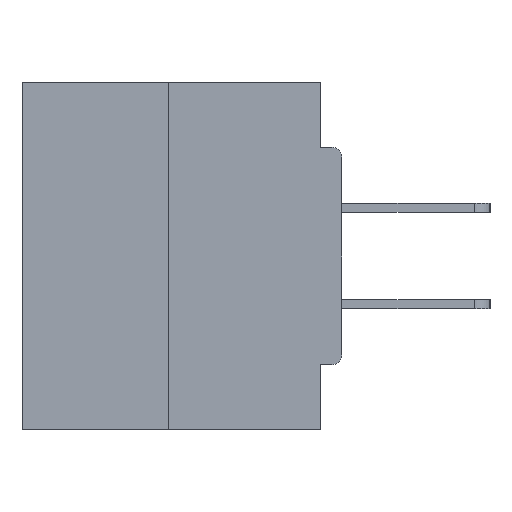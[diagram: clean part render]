
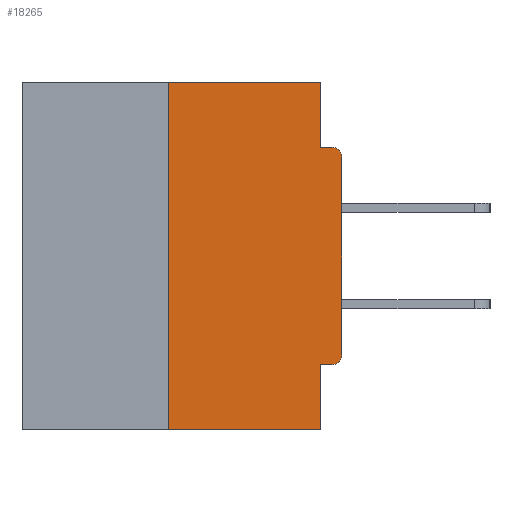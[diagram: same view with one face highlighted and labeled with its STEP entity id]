
A CAD part, left-side view. The second image highlights one B-rep face of the part: STEP entity #18265.
In plain terms, the highlighted planar face has unit normal (-1, 0, 0).
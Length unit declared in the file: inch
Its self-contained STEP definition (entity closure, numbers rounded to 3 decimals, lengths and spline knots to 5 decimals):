
#189 = CIRCLE ( 'NONE', #26565, 0.015 ) ;
#713 = DIRECTION ( 'NONE',  ( 0., -1., 0. ) ) ;
#1690 = CARTESIAN_POINT ( 'NONE',  ( 0., 0.25, 0. ) ) ;
#2110 = CARTESIAN_POINT ( 'NONE',  ( 0., 0.015, -0.0935 ) ) ;
#2321 = PLANE ( 'NONE',  #33226 ) ;
#3088 = EDGE_CURVE ( 'NONE', #15137, #19383, #21473, .T. ) ;
#3170 = VECTOR ( 'NONE', #7702, 39.37008 ) ;
#3709 = EDGE_CURVE ( 'NONE', #34003, #10903, #13700, .T. ) ;
#3812 = LINE ( 'NONE', #26926, #5011 ) ;
#3874 = FACE_OUTER_BOUND ( 'NONE', #22107, .T. ) ;
#4097 = VERTEX_POINT ( 'NONE', #36833 ) ;
#5011 = VECTOR ( 'NONE', #15619, 39.37008 ) ;
#5798 = ORIENTED_EDGE ( 'NONE', *, *, #3088, .T. ) ;
#5903 = CARTESIAN_POINT ( 'NONE',  ( 0., 0.031, -0.0935 ) ) ;
#6311 = ORIENTED_EDGE ( 'NONE', *, *, #34762, .F. ) ;
#6889 = EDGE_CURVE ( 'NONE', #4097, #21827, #26237, .T. ) ;
#7395 = CARTESIAN_POINT ( 'NONE',  ( 0., 0.031, 0. ) ) ;
#7702 = DIRECTION ( 'NONE',  ( 0., 0., -1. ) ) ;
#8331 = DIRECTION ( 'NONE',  ( 0., -1., 0. ) ) ;
#9261 = VECTOR ( 'NONE', #12833, 39.37008 ) ;
#9352 = VECTOR ( 'NONE', #18344, 39.37008 ) ;
#9856 = EDGE_CURVE ( 'NONE', #36830, #34388, #17073, .T. ) ;
#10114 = ORIENTED_EDGE ( 'NONE', *, *, #35136, .F. ) ;
#10213 = VERTEX_POINT ( 'NONE', #5903 ) ;
#10623 = DIRECTION ( 'NONE',  ( -1., 0., 0. ) ) ;
#10903 = VERTEX_POINT ( 'NONE', #17079 ) ;
#12833 = DIRECTION ( 'NONE',  ( 0., 0., 1. ) ) ;
#13700 = LINE ( 'NONE', #22921, #20709 ) ;
#14640 = VECTOR ( 'NONE', #8331, 39.37008 ) ;
#15137 = VERTEX_POINT ( 'NONE', #26985 ) ;
#15343 = DIRECTION ( 'NONE',  ( 0., 0., -1. ) ) ;
#15368 = DIRECTION ( 'NONE',  ( -1., 0., 0. ) ) ;
#15536 = CARTESIAN_POINT ( 'NONE',  ( 0., 0.015, -0.1085 ) ) ;
#15619 = DIRECTION ( 'NONE',  ( 0., -1., 0. ) ) ;
#16595 = DIRECTION ( 'NONE',  ( 1., 0., 0. ) ) ;
#17073 = LINE ( 'NONE', #23448, #28855 ) ;
#17079 = CARTESIAN_POINT ( 'NONE',  ( 0., 0.031, -0.4065 ) ) ;
#17421 = ORIENTED_EDGE ( 'NONE', *, *, #31207, .T. ) ;
#18091 = CARTESIAN_POINT ( 'NONE',  ( 0., 0.25, -0.5 ) ) ;
#18139 = LINE ( 'NONE', #29665, #9352 ) ;
#18265 = ADVANCED_FACE ( 'NONE', ( #3874 ), #2321, .F. ) ;
#18344 = DIRECTION ( 'NONE',  ( 0., 0., -1. ) ) ;
#18444 = ORIENTED_EDGE ( 'NONE', *, *, #3709, .F. ) ;
#18521 = DIRECTION ( 'NONE',  ( 0., 0., -1. ) ) ;
#18639 = CARTESIAN_POINT ( 'NONE',  ( 0., 0.031, -0.5 ) ) ;
#19141 = ORIENTED_EDGE ( 'NONE', *, *, #22095, .F. ) ;
#19383 = VERTEX_POINT ( 'NONE', #24629 ) ;
#19655 = DIRECTION ( 'NONE',  ( 0., 0., -1. ) ) ;
#19915 = CARTESIAN_POINT ( 'NONE',  ( 0., 0.031, -0.5 ) ) ;
#20709 = VECTOR ( 'NONE', #25025, 39.37008 ) ;
#20898 = EDGE_CURVE ( 'NONE', #10903, #34388, #31410, .T. ) ;
#21473 = LINE ( 'NONE', #21650, #9261 ) ;
#21650 = CARTESIAN_POINT ( 'NONE',  ( 0., 0., 0. ) ) ;
#21827 = VERTEX_POINT ( 'NONE', #7395 ) ;
#21918 = CARTESIAN_POINT ( 'NONE',  ( 0., 0.015, -0.4065 ) ) ;
#22095 = EDGE_CURVE ( 'NONE', #10213, #29325, #3812, .T. ) ;
#22107 = EDGE_LOOP ( 'NONE', ( #29617, #6311, #22419, #35456, #18444, #24707, #5798, #17421, #19141, #10114 ) ) ;
#22419 = ORIENTED_EDGE ( 'NONE', *, *, #9856, .T. ) ;
#22921 = CARTESIAN_POINT ( 'NONE',  ( 0., 0., -0.4065 ) ) ;
#23448 = CARTESIAN_POINT ( 'NONE',  ( 0., 0.46, -0.5 ) ) ;
#23788 = VECTOR ( 'NONE', #31014, 39.37008 ) ;
#24629 = CARTESIAN_POINT ( 'NONE',  ( 0., 0., -0.1085 ) ) ;
#24707 = ORIENTED_EDGE ( 'NONE', *, *, #25535, .T. ) ;
#24764 = AXIS2_PLACEMENT_3D ( 'NONE', #15536, #15368, #18521 ) ;
#25025 = DIRECTION ( 'NONE',  ( 0., 1., 0. ) ) ;
#25152 = LINE ( 'NONE', #1690, #23788 ) ;
#25535 = EDGE_CURVE ( 'NONE', #34003, #15137, #189, .T. ) ;
#26237 = LINE ( 'NONE', #34688, #14640 ) ;
#26565 = AXIS2_PLACEMENT_3D ( 'NONE', #33564, #10623, #19655 ) ;
#26926 = CARTESIAN_POINT ( 'NONE',  ( 0., 0., -0.0935 ) ) ;
#26985 = CARTESIAN_POINT ( 'NONE',  ( 0., 0., -0.3915 ) ) ;
#27776 = CIRCLE ( 'NONE', #24764, 0.015 ) ;
#28855 = VECTOR ( 'NONE', #713, 39.37008 ) ;
#29325 = VERTEX_POINT ( 'NONE', #2110 ) ;
#29617 = ORIENTED_EDGE ( 'NONE', *, *, #6889, .F. ) ;
#29665 = CARTESIAN_POINT ( 'NONE',  ( 0., 0.031, 0. ) ) ;
#31014 = DIRECTION ( 'NONE',  ( 0., 0., 1. ) ) ;
#31207 = EDGE_CURVE ( 'NONE', #19383, #29325, #27776, .T. ) ;
#31410 = LINE ( 'NONE', #19915, #3170 ) ;
#33189 = CARTESIAN_POINT ( 'NONE',  ( 0., 0.46, 0. ) ) ;
#33226 = AXIS2_PLACEMENT_3D ( 'NONE', #33189, #16595, #15343 ) ;
#33564 = CARTESIAN_POINT ( 'NONE',  ( 0., 0.015, -0.3915 ) ) ;
#34003 = VERTEX_POINT ( 'NONE', #21918 ) ;
#34388 = VERTEX_POINT ( 'NONE', #18639 ) ;
#34688 = CARTESIAN_POINT ( 'NONE',  ( 0., 0.46, 0. ) ) ;
#34762 = EDGE_CURVE ( 'NONE', #36830, #4097, #25152, .T. ) ;
#35136 = EDGE_CURVE ( 'NONE', #21827, #10213, #18139, .T. ) ;
#35456 = ORIENTED_EDGE ( 'NONE', *, *, #20898, .F. ) ;
#36830 = VERTEX_POINT ( 'NONE', #18091 ) ;
#36833 = CARTESIAN_POINT ( 'NONE',  ( 0., 0.25, 0. ) ) ;
